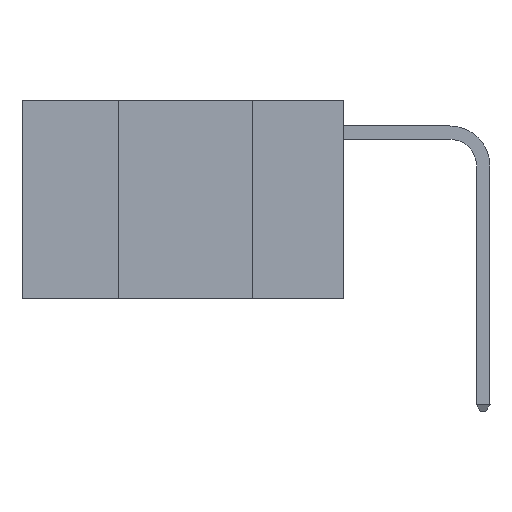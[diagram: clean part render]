
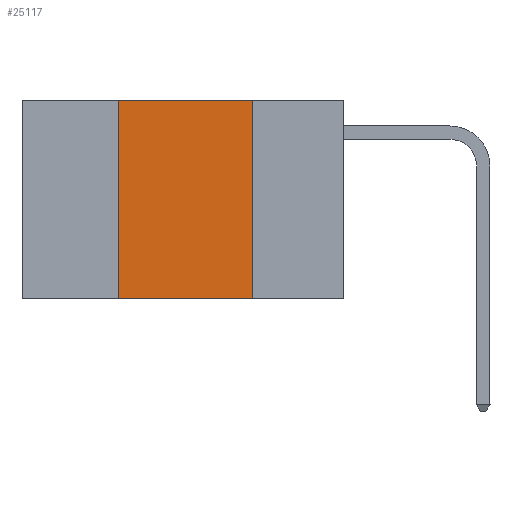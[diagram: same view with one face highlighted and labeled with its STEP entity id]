
A CAD part, left-side view. The second image highlights one B-rep face of the part: STEP entity #25117.
In plain terms, the highlighted planar face has unit normal (-1, 0, 0).
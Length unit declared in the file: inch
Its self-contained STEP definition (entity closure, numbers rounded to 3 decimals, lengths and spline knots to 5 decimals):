
#308 = CARTESIAN_POINT ( 'NONE',  ( 0., 0.6, -0.37 ) ) ;
#881 = EDGE_CURVE ( 'NONE', #16320, #3704, #24594, .T. ) ;
#2339 = VECTOR ( 'NONE', #26269, 39.37008 ) ;
#3704 = VERTEX_POINT ( 'NONE', #23546 ) ;
#3855 = CARTESIAN_POINT ( 'NONE',  ( 0., 0.42, -0.37 ) ) ;
#4770 = DIRECTION ( 'NONE',  ( 0., 0., -1. ) ) ;
#6393 = CARTESIAN_POINT ( 'NONE',  ( 0., 0.42, 0. ) ) ;
#6449 = EDGE_CURVE ( 'NONE', #16320, #26322, #18369, .T. ) ;
#7095 = DIRECTION ( 'NONE',  ( 1., 0., 0. ) ) ;
#7217 = LINE ( 'NONE', #15075, #23018 ) ;
#8715 = DIRECTION ( 'NONE',  ( 0., -1., 0. ) ) ;
#11778 = FACE_OUTER_BOUND ( 'NONE', #13388, .T. ) ;
#13033 = VECTOR ( 'NONE', #8715, 39.37008 ) ;
#13119 = PLANE ( 'NONE',  #24116 ) ;
#13388 = EDGE_LOOP ( 'NONE', ( #22207, #22798, #22910, #23164 ) ) ;
#15075 = CARTESIAN_POINT ( 'NONE',  ( 0., 0.17, 0. ) ) ;
#16320 = VERTEX_POINT ( 'NONE', #3855 ) ;
#16962 = EDGE_CURVE ( 'NONE', #26322, #22590, #24297, .T. ) ;
#17715 = VECTOR ( 'NONE', #24461, 39.37008 ) ;
#18369 = LINE ( 'NONE', #26058, #17715 ) ;
#19424 = CARTESIAN_POINT ( 'NONE',  ( 0., 0.6, 0. ) ) ;
#20379 = CARTESIAN_POINT ( 'NONE',  ( 0., 0.17, 0. ) ) ;
#21514 = DIRECTION ( 'NONE',  ( 0., 0., -1. ) ) ;
#22207 = ORIENTED_EDGE ( 'NONE', *, *, #25728, .F. ) ;
#22590 = VERTEX_POINT ( 'NONE', #20379 ) ;
#22798 = ORIENTED_EDGE ( 'NONE', *, *, #16962, .F. ) ;
#22910 = ORIENTED_EDGE ( 'NONE', *, *, #6449, .F. ) ;
#23018 = VECTOR ( 'NONE', #4770, 39.37008 ) ;
#23164 = ORIENTED_EDGE ( 'NONE', *, *, #881, .T. ) ;
#23546 = CARTESIAN_POINT ( 'NONE',  ( 0., 0.17, -0.37 ) ) ;
#24116 = AXIS2_PLACEMENT_3D ( 'NONE', #19424, #7095, #21514 ) ;
#24225 = CARTESIAN_POINT ( 'NONE',  ( 0., 0.6, 0. ) ) ;
#24297 = LINE ( 'NONE', #24225, #2339 ) ;
#24461 = DIRECTION ( 'NONE',  ( 0., 0., 1. ) ) ;
#24594 = LINE ( 'NONE', #308, #13033 ) ;
#25117 = ADVANCED_FACE ( 'NONE', ( #11778 ), #13119, .F. ) ;
#25728 = EDGE_CURVE ( 'NONE', #22590, #3704, #7217, .T. ) ;
#26058 = CARTESIAN_POINT ( 'NONE',  ( 0., 0.42, 0. ) ) ;
#26269 = DIRECTION ( 'NONE',  ( 0., -1., 0. ) ) ;
#26322 = VERTEX_POINT ( 'NONE', #6393 ) ;
